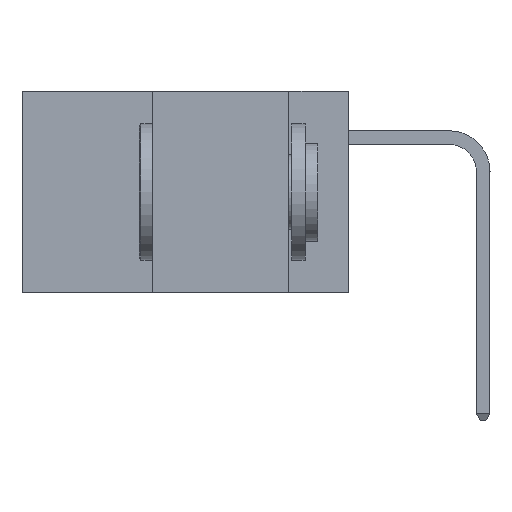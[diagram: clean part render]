
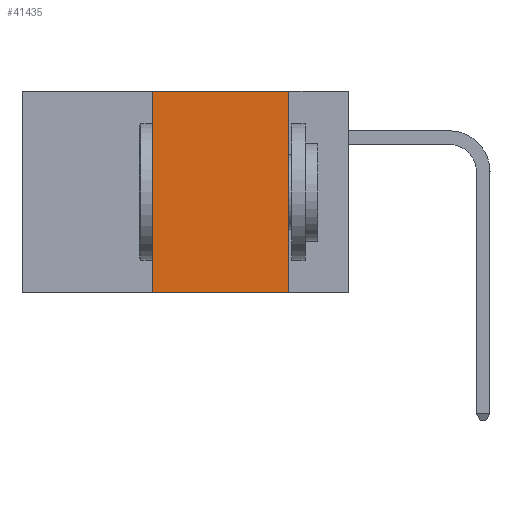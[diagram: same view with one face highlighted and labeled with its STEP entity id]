
A CAD part, left-side view. The second image highlights one B-rep face of the part: STEP entity #41435.
In plain terms, the highlighted planar face has unit normal (-1, 0, 0).
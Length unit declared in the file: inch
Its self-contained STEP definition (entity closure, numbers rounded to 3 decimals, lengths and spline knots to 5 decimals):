
#2917 = VERTEX_POINT ( 'NONE', #16453 ) ;
#3582 = CARTESIAN_POINT ( 'NONE',  ( 0., 0.6, 0. ) ) ;
#4944 = CARTESIAN_POINT ( 'NONE',  ( 0., 0.11, 0. ) ) ;
#6805 = LINE ( 'NONE', #19714, #32658 ) ;
#7211 = CARTESIAN_POINT ( 'NONE',  ( 0., 0.11, 0. ) ) ;
#7265 = AXIS2_PLACEMENT_3D ( 'NONE', #15822, #12544, #36096 ) ;
#7656 = FACE_OUTER_BOUND ( 'NONE', #18726, .T. ) ;
#8386 = ORIENTED_EDGE ( 'NONE', *, *, #11414, .T. ) ;
#11414 = EDGE_CURVE ( 'NONE', #2917, #37455, #13235, .T. ) ;
#12544 = DIRECTION ( 'NONE',  ( 1., 0., 0. ) ) ;
#13235 = LINE ( 'NONE', #37936, #21151 ) ;
#14421 = DIRECTION ( 'NONE',  ( 0., -1., 0. ) ) ;
#15822 = CARTESIAN_POINT ( 'NONE',  ( 0., 0.6, 0. ) ) ;
#16453 = CARTESIAN_POINT ( 'NONE',  ( 0., 0.36, -0.37 ) ) ;
#16574 = VERTEX_POINT ( 'NONE', #27927 ) ;
#17206 = DIRECTION ( 'NONE',  ( 0., -1., 0. ) ) ;
#18225 = EDGE_CURVE ( 'NONE', #2917, #16574, #6805, .T. ) ;
#18659 = VECTOR ( 'NONE', #42015, 39.37008 ) ;
#18726 = EDGE_LOOP ( 'NONE', ( #26937, #31205, #31424, #8386 ) ) ;
#19714 = CARTESIAN_POINT ( 'NONE',  ( 0., 0.36, 0. ) ) ;
#21151 = VECTOR ( 'NONE', #14421, 39.37008 ) ;
#22008 = VERTEX_POINT ( 'NONE', #7211 ) ;
#26453 = DIRECTION ( 'NONE',  ( 0., 0., 1. ) ) ;
#26937 = ORIENTED_EDGE ( 'NONE', *, *, #36227, .F. ) ;
#27570 = LINE ( 'NONE', #4944, #18659 ) ;
#27927 = CARTESIAN_POINT ( 'NONE',  ( 0., 0.36, 0. ) ) ;
#28687 = EDGE_CURVE ( 'NONE', #16574, #22008, #42513, .T. ) ;
#31205 = ORIENTED_EDGE ( 'NONE', *, *, #28687, .F. ) ;
#31424 = ORIENTED_EDGE ( 'NONE', *, *, #18225, .F. ) ;
#32658 = VECTOR ( 'NONE', #26453, 39.37008 ) ;
#33621 = VECTOR ( 'NONE', #17206, 39.37008 ) ;
#34918 = CARTESIAN_POINT ( 'NONE',  ( 0., 0.11, -0.37 ) ) ;
#36096 = DIRECTION ( 'NONE',  ( 0., 0., -1. ) ) ;
#36227 = EDGE_CURVE ( 'NONE', #22008, #37455, #27570, .T. ) ;
#37455 = VERTEX_POINT ( 'NONE', #34918 ) ;
#37936 = CARTESIAN_POINT ( 'NONE',  ( 0., 0.6, -0.37 ) ) ;
#39302 = PLANE ( 'NONE',  #7265 ) ;
#41435 = ADVANCED_FACE ( 'NONE', ( #7656 ), #39302, .F. ) ;
#42015 = DIRECTION ( 'NONE',  ( 0., 0., -1. ) ) ;
#42513 = LINE ( 'NONE', #3582, #33621 ) ;
